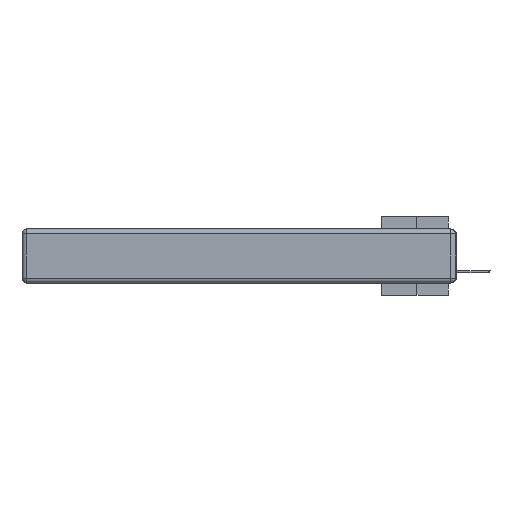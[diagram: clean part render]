
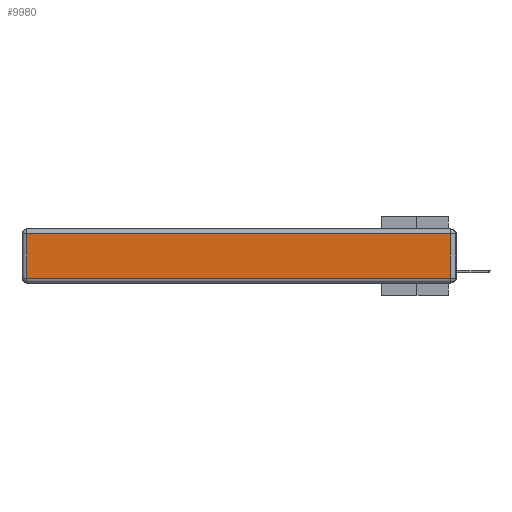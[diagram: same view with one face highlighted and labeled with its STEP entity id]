
A CAD part, left-side view. The second image highlights one B-rep face of the part: STEP entity #9980.
In plain terms, the highlighted planar face has unit normal (-1, 0, 0).
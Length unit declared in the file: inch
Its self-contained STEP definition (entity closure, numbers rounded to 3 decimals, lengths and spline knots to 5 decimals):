
#709 = VERTEX_POINT ( 'NONE', #6860 ) ;
#1197 = ORIENTED_EDGE ( 'NONE', *, *, #16549, .T. ) ;
#1230 = VECTOR ( 'NONE', #16932, 39.37008 ) ;
#2684 = LINE ( 'NONE', #5296, #1230 ) ;
#2726 = DIRECTION ( 'NONE',  ( 0., 0., 1. ) ) ;
#4849 = DIRECTION ( 'NONE',  ( 0., -1., 0. ) ) ;
#5015 = VERTEX_POINT ( 'NONE', #10038 ) ;
#5232 = CARTESIAN_POINT ( 'NONE',  ( 0., 0.03, -0.343 ) ) ;
#5296 = CARTESIAN_POINT ( 'NONE',  ( 0., 2.75, -0.03 ) ) ;
#5435 = EDGE_CURVE ( 'NONE', #5015, #22559, #6780, .T. ) ;
#5744 = LINE ( 'NONE', #5232, #26753 ) ;
#6780 = LINE ( 'NONE', #8818, #10760 ) ;
#6860 = CARTESIAN_POINT ( 'NONE',  ( 0., 0.03, -0.03 ) ) ;
#7138 = CARTESIAN_POINT ( 'NONE',  ( 0., 0., -0.313 ) ) ;
#7551 = DIRECTION ( 'NONE',  ( 0., 0., 1. ) ) ;
#8818 = CARTESIAN_POINT ( 'NONE',  ( 0., 2.72, -0.343 ) ) ;
#9165 = ORIENTED_EDGE ( 'NONE', *, *, #19403, .T. ) ;
#9980 = ADVANCED_FACE ( 'NONE', ( #17364 ), #16450, .T. ) ;
#10038 = CARTESIAN_POINT ( 'NONE',  ( 0., 2.72, -0.03 ) ) ;
#10760 = VECTOR ( 'NONE', #29353, 39.37008 ) ;
#11769 = DIRECTION ( 'NONE',  ( -1., 0., 0. ) ) ;
#14304 = ORIENTED_EDGE ( 'NONE', *, *, #5435, .T. ) ;
#14503 = CARTESIAN_POINT ( 'NONE',  ( 0., 0., -0.343 ) ) ;
#16450 = PLANE ( 'NONE',  #25581 ) ;
#16549 = EDGE_CURVE ( 'NONE', #18851, #709, #5744, .T. ) ;
#16896 = CARTESIAN_POINT ( 'NONE',  ( 0., 2.72, -0.313 ) ) ;
#16932 = DIRECTION ( 'NONE',  ( 0., 1., 0. ) ) ;
#17364 = FACE_OUTER_BOUND ( 'NONE', #26808, .T. ) ;
#18851 = VERTEX_POINT ( 'NONE', #19376 ) ;
#19376 = CARTESIAN_POINT ( 'NONE',  ( 0., 0.03, -0.313 ) ) ;
#19403 = EDGE_CURVE ( 'NONE', #709, #5015, #2684, .T. ) ;
#20641 = LINE ( 'NONE', #7138, #25714 ) ;
#22559 = VERTEX_POINT ( 'NONE', #16896 ) ;
#24628 = ORIENTED_EDGE ( 'NONE', *, *, #24907, .T. ) ;
#24907 = EDGE_CURVE ( 'NONE', #22559, #18851, #20641, .T. ) ;
#25581 = AXIS2_PLACEMENT_3D ( 'NONE', #14503, #11769, #2726 ) ;
#25714 = VECTOR ( 'NONE', #4849, 39.37008 ) ;
#26753 = VECTOR ( 'NONE', #7551, 39.37008 ) ;
#26808 = EDGE_LOOP ( 'NONE', ( #24628, #1197, #9165, #14304 ) ) ;
#29353 = DIRECTION ( 'NONE',  ( 0., 0., -1. ) ) ;
